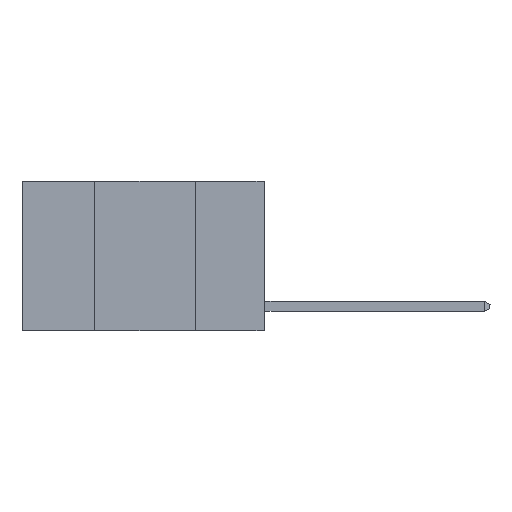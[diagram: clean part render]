
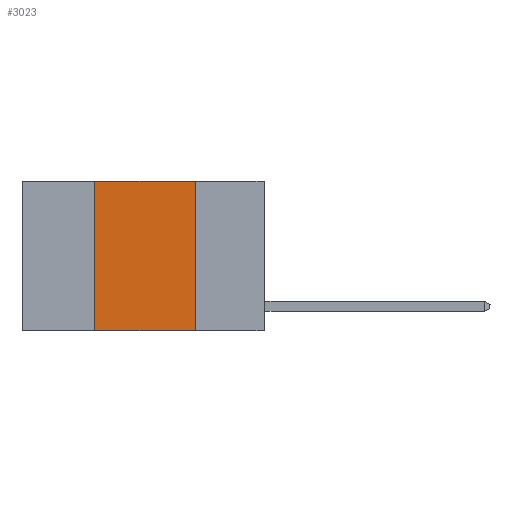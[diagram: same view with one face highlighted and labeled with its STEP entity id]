
A CAD part, left-side view. The second image highlights one B-rep face of the part: STEP entity #3023.
In plain terms, the highlighted planar face has unit normal (-1, 0, 0).
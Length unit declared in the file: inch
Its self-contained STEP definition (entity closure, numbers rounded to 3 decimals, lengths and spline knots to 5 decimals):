
#310 = DIRECTION ( 'NONE',  ( 0., 0., 1. ) ) ;
#533 = LINE ( 'NONE', #1315, #10842 ) ;
#779 = ORIENTED_EDGE ( 'NONE', *, *, #9216, .F. ) ;
#1315 = CARTESIAN_POINT ( 'NONE',  ( 0., 0.42, 0. ) ) ;
#1752 = LINE ( 'NONE', #5292, #4768 ) ;
#2046 = EDGE_CURVE ( 'NONE', #9813, #3798, #533, .T. ) ;
#2230 = CARTESIAN_POINT ( 'NONE',  ( 0., 0.6, 0. ) ) ;
#2532 = ORIENTED_EDGE ( 'NONE', *, *, #8073, .F. ) ;
#3023 = ADVANCED_FACE ( 'NONE', ( #3637 ), #7607, .F. ) ;
#3188 = EDGE_CURVE ( 'NONE', #9813, #8964, #1752, .T. ) ;
#3457 = VECTOR ( 'NONE', #9273, 39.37008 ) ;
#3637 = FACE_OUTER_BOUND ( 'NONE', #7501, .T. ) ;
#3693 = CARTESIAN_POINT ( 'NONE',  ( 0., 0.42, 0. ) ) ;
#3798 = VERTEX_POINT ( 'NONE', #3693 ) ;
#4481 = CARTESIAN_POINT ( 'NONE',  ( 0., 0.17, -0.37 ) ) ;
#4768 = VECTOR ( 'NONE', #6161, 39.37008 ) ;
#5292 = CARTESIAN_POINT ( 'NONE',  ( 0., 0.6, -0.37 ) ) ;
#5536 = ORIENTED_EDGE ( 'NONE', *, *, #3188, .T. ) ;
#5601 = LINE ( 'NONE', #6802, #3457 ) ;
#6161 = DIRECTION ( 'NONE',  ( 0., -1., 0. ) ) ;
#6445 = DIRECTION ( 'NONE',  ( 0., 0., -1. ) ) ;
#6572 = VERTEX_POINT ( 'NONE', #11746 ) ;
#6802 = CARTESIAN_POINT ( 'NONE',  ( 0., 0.6, 0. ) ) ;
#7501 = EDGE_LOOP ( 'NONE', ( #2532, #779, #8706, #5536 ) ) ;
#7607 = PLANE ( 'NONE',  #10844 ) ;
#7734 = DIRECTION ( 'NONE',  ( 0., 0., -1. ) ) ;
#7766 = DIRECTION ( 'NONE',  ( 1., 0., 0. ) ) ;
#8073 = EDGE_CURVE ( 'NONE', #6572, #8964, #8909, .T. ) ;
#8562 = CARTESIAN_POINT ( 'NONE',  ( 0., 0.42, -0.37 ) ) ;
#8706 = ORIENTED_EDGE ( 'NONE', *, *, #2046, .F. ) ;
#8909 = LINE ( 'NONE', #10019, #11620 ) ;
#8964 = VERTEX_POINT ( 'NONE', #4481 ) ;
#9216 = EDGE_CURVE ( 'NONE', #3798, #6572, #5601, .T. ) ;
#9273 = DIRECTION ( 'NONE',  ( 0., -1., 0. ) ) ;
#9813 = VERTEX_POINT ( 'NONE', #8562 ) ;
#10019 = CARTESIAN_POINT ( 'NONE',  ( 0., 0.17, 0. ) ) ;
#10842 = VECTOR ( 'NONE', #310, 39.37008 ) ;
#10844 = AXIS2_PLACEMENT_3D ( 'NONE', #2230, #7766, #7734 ) ;
#11620 = VECTOR ( 'NONE', #6445, 39.37008 ) ;
#11746 = CARTESIAN_POINT ( 'NONE',  ( 0., 0.17, 0. ) ) ;
